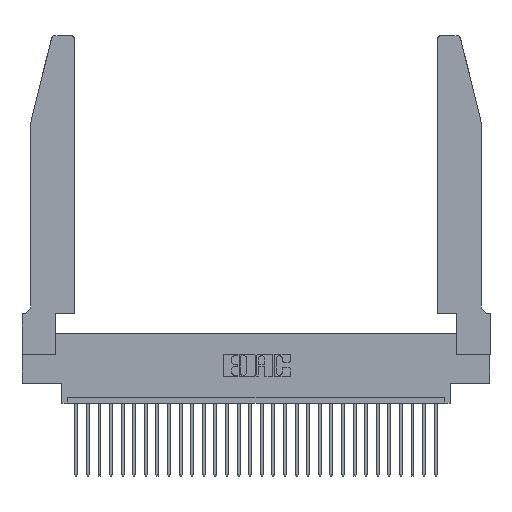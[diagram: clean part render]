
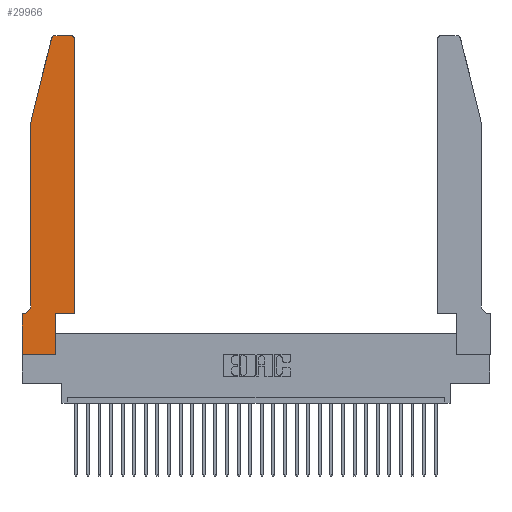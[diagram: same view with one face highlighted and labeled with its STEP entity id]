
A CAD part, top view. The second image highlights one B-rep face of the part: STEP entity #29966.
In plain terms, the highlighted planar face has unit normal (0, 0, 1).
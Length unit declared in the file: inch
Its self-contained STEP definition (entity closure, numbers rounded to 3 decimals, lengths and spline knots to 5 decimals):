
#464 = CARTESIAN_POINT ( 'NONE',  ( 0.4505, 0.35, 0.37 ) ) ;
#511 = VERTEX_POINT ( 'NONE', #3027 ) ;
#1456 = ORIENTED_EDGE ( 'NONE', *, *, #27567, .T. ) ;
#1464 = DIRECTION ( 'NONE',  ( 1., 0., 0. ) ) ;
#1562 = ORIENTED_EDGE ( 'NONE', *, *, #5111, .T. ) ;
#1620 = VECTOR ( 'NONE', #8647, 39.37008 ) ;
#2056 = CARTESIAN_POINT ( 'NONE',  ( 0.0055, 0.42, 0.37 ) ) ;
#2571 = EDGE_CURVE ( 'NONE', #10814, #19368, #21721, .T. ) ;
#3027 = CARTESIAN_POINT ( 'NONE',  ( 0.0755, 0.42, 0.37 ) ) ;
#3500 = LINE ( 'NONE', #21852, #25454 ) ;
#4146 = EDGE_CURVE ( 'NONE', #19368, #13526, #23484, .T. ) ;
#4446 = DIRECTION ( 'NONE',  ( -1., 0., 0. ) ) ;
#4582 = CARTESIAN_POINT ( 'NONE',  ( 0.0055, 0.35, 0.37 ) ) ;
#4762 = CARTESIAN_POINT ( 'NONE',  ( 0.0755, 0.35, 0.37 ) ) ;
#5111 = EDGE_CURVE ( 'NONE', #13526, #17220, #23423, .T. ) ;
#5184 = VECTOR ( 'NONE', #20893, 39.37008 ) ;
#5815 = CARTESIAN_POINT ( 'NONE',  ( 0.2865, 0., 0.37 ) ) ;
#6196 = CARTESIAN_POINT ( 'NONE',  ( 0.0755, 2., 0.37 ) ) ;
#6780 = LINE ( 'NONE', #22332, #27655 ) ;
#6859 = VERTEX_POINT ( 'NONE', #19010 ) ;
#7337 = DIRECTION ( 'NONE',  ( 1., 0., 0. ) ) ;
#7519 = ORIENTED_EDGE ( 'NONE', *, *, #28537, .T. ) ;
#7763 = DIRECTION ( 'NONE',  ( 0., 0., 1. ) ) ;
#7854 = CIRCLE ( 'NONE', #25646, 0.07 ) ;
#7929 = VECTOR ( 'NONE', #21514, 39.37008 ) ;
#7937 = EDGE_CURVE ( 'NONE', #18871, #6859, #3500, .T. ) ;
#8000 = CARTESIAN_POINT ( 'NONE',  ( 0.4505, 0.35, 0.37 ) ) ;
#8343 = CARTESIAN_POINT ( 'NONE',  ( 0., 0.35, 0.37 ) ) ;
#8647 = DIRECTION ( 'NONE',  ( -0.239, -0.971, 0. ) ) ;
#8865 = ORIENTED_EDGE ( 'NONE', *, *, #28966, .T. ) ;
#9343 = EDGE_CURVE ( 'NONE', #27205, #26163, #13338, .T. ) ;
#10128 = CARTESIAN_POINT ( 'NONE',  ( 0.25487, 2.72718, 0.37 ) ) ;
#10296 = ORIENTED_EDGE ( 'NONE', *, *, #9343, .T. ) ;
#10299 = VECTOR ( 'NONE', #28940, 39.37008 ) ;
#10539 = ORIENTED_EDGE ( 'NONE', *, *, #2571, .T. ) ;
#10814 = VERTEX_POINT ( 'NONE', #18093 ) ;
#11694 = VERTEX_POINT ( 'NONE', #19624 ) ;
#12919 = VECTOR ( 'NONE', #14605, 39.37008 ) ;
#13139 = DIRECTION ( 'NONE',  ( 0., 0., 1. ) ) ;
#13338 = LINE ( 'NONE', #25131, #1620 ) ;
#13526 = VERTEX_POINT ( 'NONE', #23115 ) ;
#14332 = EDGE_CURVE ( 'NONE', #26163, #511, #21128, .T. ) ;
#14439 = CARTESIAN_POINT ( 'NONE',  ( 0.284, 2.72, 0.37 ) ) ;
#14605 = DIRECTION ( 'NONE',  ( 1., 0., 0. ) ) ;
#14700 = ORIENTED_EDGE ( 'NONE', *, *, #4146, .T. ) ;
#16255 = CARTESIAN_POINT ( 'NONE',  ( 0.2865, 0.35, 0.37 ) ) ;
#16486 = ORIENTED_EDGE ( 'NONE', *, *, #17709, .T. ) ;
#16782 = CARTESIAN_POINT ( 'NONE',  ( 0., 0.35, 0.37 ) ) ;
#17054 = ORIENTED_EDGE ( 'NONE', *, *, #14332, .T. ) ;
#17133 = EDGE_CURVE ( 'NONE', #22168, #10814, #25343, .T. ) ;
#17220 = VERTEX_POINT ( 'NONE', #24402 ) ;
#17709 = EDGE_CURVE ( 'NONE', #25326, #18871, #21256, .T. ) ;
#18093 = CARTESIAN_POINT ( 'NONE',  ( 0.2865, 0.35, 0.37 ) ) ;
#18436 = DIRECTION ( 'NONE',  ( 0., 0., -1. ) ) ;
#18623 = DIRECTION ( 'NONE',  ( 0., 1., 0. ) ) ;
#18773 = AXIS2_PLACEMENT_3D ( 'NONE', #14439, #7763, #19153 ) ;
#18804 = EDGE_CURVE ( 'NONE', #11694, #27205, #25221, .T. ) ;
#18871 = VERTEX_POINT ( 'NONE', #16782 ) ;
#19010 = CARTESIAN_POINT ( 'NONE',  ( 0., 0., 0.37 ) ) ;
#19097 = DIRECTION ( 'NONE',  ( 0., -1., 0. ) ) ;
#19153 = DIRECTION ( 'NONE',  ( 1., 0., 0. ) ) ;
#19160 = CARTESIAN_POINT ( 'NONE',  ( 0.0755, 2., 0.37 ) ) ;
#19368 = VERTEX_POINT ( 'NONE', #28719 ) ;
#19624 = CARTESIAN_POINT ( 'NONE',  ( 0.284, 2.75, 0.37 ) ) ;
#19809 = ORIENTED_EDGE ( 'NONE', *, *, #18804, .T. ) ;
#20112 = CARTESIAN_POINT ( 'NONE',  ( 0.4205, 2.72, 0.37 ) ) ;
#20893 = DIRECTION ( 'NONE',  ( -1., 0., 0. ) ) ;
#21128 = LINE ( 'NONE', #19160, #7929 ) ;
#21143 = VECTOR ( 'NONE', #7337, 39.37008 ) ;
#21256 = LINE ( 'NONE', #4762, #5184 ) ;
#21514 = DIRECTION ( 'NONE',  ( 0., -1., 0. ) ) ;
#21721 = LINE ( 'NONE', #464, #12919 ) ;
#21729 = AXIS2_PLACEMENT_3D ( 'NONE', #8343, #13139, #1464 ) ;
#21852 = CARTESIAN_POINT ( 'NONE',  ( 0., 0., 0.37 ) ) ;
#22051 = VECTOR ( 'NONE', #18623, 39.37008 ) ;
#22168 = VERTEX_POINT ( 'NONE', #5815 ) ;
#22332 = CARTESIAN_POINT ( 'NONE',  ( 0.2605, 2.75, 0.37 ) ) ;
#23115 = CARTESIAN_POINT ( 'NONE',  ( 0.4505, 2.72, 0.37 ) ) ;
#23142 = ORIENTED_EDGE ( 'NONE', *, *, #17133, .T. ) ;
#23423 = CIRCLE ( 'NONE', #27618, 0.03 ) ;
#23484 = LINE ( 'NONE', #8000, #10299 ) ;
#24402 = CARTESIAN_POINT ( 'NONE',  ( 0.4205, 2.75, 0.37 ) ) ;
#24690 = DIRECTION ( 'NONE',  ( -1., 0., 0. ) ) ;
#24835 = PLANE ( 'NONE',  #21729 ) ;
#25131 = CARTESIAN_POINT ( 'NONE',  ( 0.0755, 2., 0.37 ) ) ;
#25221 = CIRCLE ( 'NONE', #18773, 0.03 ) ;
#25230 = DIRECTION ( 'NONE',  ( 0., 0., 1. ) ) ;
#25326 = VERTEX_POINT ( 'NONE', #4582 ) ;
#25343 = LINE ( 'NONE', #16255, #22051 ) ;
#25454 = VECTOR ( 'NONE', #19097, 39.37008 ) ;
#25525 = LINE ( 'NONE', #28411, #21143 ) ;
#25646 = AXIS2_PLACEMENT_3D ( 'NONE', #2056, #18436, #4446 ) ;
#26163 = VERTEX_POINT ( 'NONE', #6196 ) ;
#27205 = VERTEX_POINT ( 'NONE', #10128 ) ;
#27488 = ORIENTED_EDGE ( 'NONE', *, *, #7937, .T. ) ;
#27567 = EDGE_CURVE ( 'NONE', #6859, #22168, #25525, .T. ) ;
#27576 = DIRECTION ( 'NONE',  ( 1., 0., 0. ) ) ;
#27618 = AXIS2_PLACEMENT_3D ( 'NONE', #20112, #25230, #27576 ) ;
#27655 = VECTOR ( 'NONE', #24690, 39.37008 ) ;
#28411 = CARTESIAN_POINT ( 'NONE',  ( 0., 0., 0.37 ) ) ;
#28537 = EDGE_CURVE ( 'NONE', #17220, #11694, #6780, .T. ) ;
#28633 = FACE_OUTER_BOUND ( 'NONE', #30015, .T. ) ;
#28719 = CARTESIAN_POINT ( 'NONE',  ( 0.4505, 0.35, 0.37 ) ) ;
#28940 = DIRECTION ( 'NONE',  ( 0., 1., 0. ) ) ;
#28966 = EDGE_CURVE ( 'NONE', #511, #25326, #7854, .T. ) ;
#29966 = ADVANCED_FACE ( 'NONE', ( #28633 ), #24835, .T. ) ;
#30015 = EDGE_LOOP ( 'NONE', ( #7519, #19809, #10296, #17054, #8865, #16486, #27488, #1456, #23142, #10539, #14700, #1562 ) ) ;
